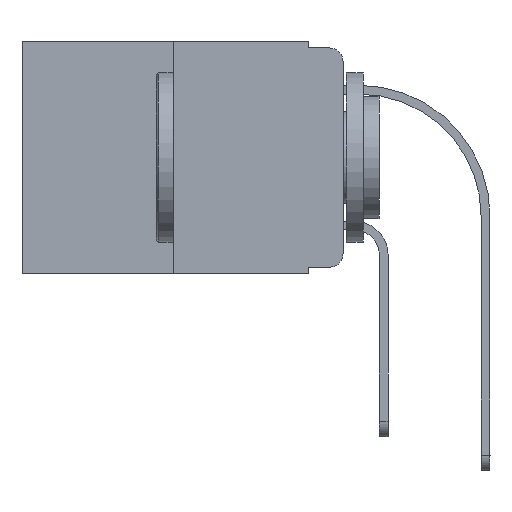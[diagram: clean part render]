
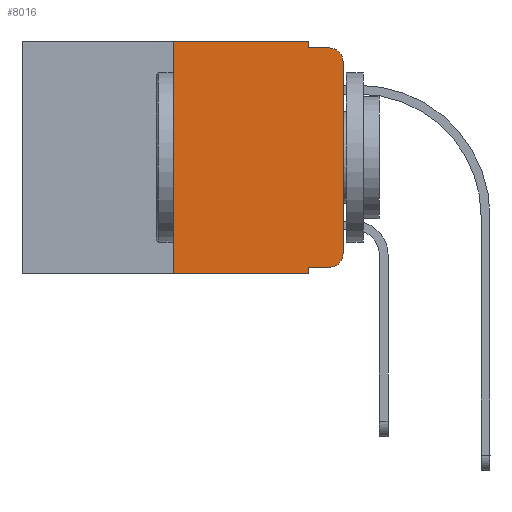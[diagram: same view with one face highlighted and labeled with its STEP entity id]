
A CAD part, left-side view. The second image highlights one B-rep face of the part: STEP entity #8016.
In plain terms, the highlighted planar face has unit normal (-1, 0, 0).
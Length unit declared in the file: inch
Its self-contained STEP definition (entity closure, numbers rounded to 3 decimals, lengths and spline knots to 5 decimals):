
#604 = ORIENTED_EDGE ( 'NONE', *, *, #14127, .T. ) ;
#701 = VERTEX_POINT ( 'NONE', #3576 ) ;
#734 = DIRECTION ( 'NONE',  ( 0., -1., 0. ) ) ;
#1061 = VECTOR ( 'NONE', #15440, 39.37008 ) ;
#1544 = VERTEX_POINT ( 'NONE', #9399 ) ;
#1588 = VECTOR ( 'NONE', #6368, 39.37008 ) ;
#1651 = CARTESIAN_POINT ( 'NONE',  ( 0., 0., 0. ) ) ;
#1813 = LINE ( 'NONE', #12721, #18763 ) ;
#1842 = EDGE_CURVE ( 'NONE', #6208, #13516, #20050, .T. ) ;
#2328 = CARTESIAN_POINT ( 'NONE',  ( 0., 0.473, 0. ) ) ;
#2438 = DIRECTION ( 'NONE',  ( 1., 0., 0. ) ) ;
#2763 = AXIS2_PLACEMENT_3D ( 'NONE', #20261, #9023, #14079 ) ;
#2826 = EDGE_LOOP ( 'NONE', ( #6298, #4714, #5255, #6037, #14143, #20571, #604, #4572, #17367, #7953 ) ) ;
#2975 = CARTESIAN_POINT ( 'NONE',  ( 0., 0.051, -0.01 ) ) ;
#3067 = LINE ( 'NONE', #9663, #14482 ) ;
#3576 = CARTESIAN_POINT ( 'NONE',  ( 0., 0.25, -0.343 ) ) ;
#4572 = ORIENTED_EDGE ( 'NONE', *, *, #15719, .F. ) ;
#4573 = EDGE_CURVE ( 'NONE', #1544, #17947, #17360, .T. ) ;
#4714 = ORIENTED_EDGE ( 'NONE', *, *, #16092, .T. ) ;
#4744 = DIRECTION ( 'NONE',  ( 0., -1., 0. ) ) ;
#4976 = LINE ( 'NONE', #14415, #9461 ) ;
#5255 = ORIENTED_EDGE ( 'NONE', *, *, #11853, .F. ) ;
#5357 = CARTESIAN_POINT ( 'NONE',  ( 0., 0.473, 0. ) ) ;
#5797 = DIRECTION ( 'NONE',  ( 0., 0., -1. ) ) ;
#5975 = EDGE_CURVE ( 'NONE', #14881, #17803, #6157, .T. ) ;
#5980 = CARTESIAN_POINT ( 'NONE',  ( 0., 0.02, -0.03 ) ) ;
#6037 = ORIENTED_EDGE ( 'NONE', *, *, #4573, .F. ) ;
#6157 = LINE ( 'NONE', #1651, #1588 ) ;
#6208 = VERTEX_POINT ( 'NONE', #13477 ) ;
#6277 = VERTEX_POINT ( 'NONE', #12013 ) ;
#6298 = ORIENTED_EDGE ( 'NONE', *, *, #5975, .T. ) ;
#6368 = DIRECTION ( 'NONE',  ( 0., 0., 1. ) ) ;
#7904 = VECTOR ( 'NONE', #15591, 39.37008 ) ;
#7953 = ORIENTED_EDGE ( 'NONE', *, *, #19572, .T. ) ;
#8016 = ADVANCED_FACE ( 'NONE', ( #12410 ), #19958, .F. ) ;
#8118 = CIRCLE ( 'NONE', #12814, 0.02 ) ;
#9023 = DIRECTION ( 'NONE',  ( -1., 0., 0. ) ) ;
#9180 = CARTESIAN_POINT ( 'NONE',  ( 0., 0.051, 0. ) ) ;
#9399 = CARTESIAN_POINT ( 'NONE',  ( 0., 0.051, 0. ) ) ;
#9461 = VECTOR ( 'NONE', #9682, 39.37008 ) ;
#9663 = CARTESIAN_POINT ( 'NONE',  ( 0., 0.051, 0. ) ) ;
#9682 = DIRECTION ( 'NONE',  ( 0., -1., 0. ) ) ;
#10617 = CARTESIAN_POINT ( 'NONE',  ( 0., 0.051, -0.333 ) ) ;
#11186 = DIRECTION ( 'NONE',  ( 0., 0., 1. ) ) ;
#11853 = EDGE_CURVE ( 'NONE', #17947, #14939, #1813, .T. ) ;
#12013 = CARTESIAN_POINT ( 'NONE',  ( 0., 0.25, 0. ) ) ;
#12074 = EDGE_CURVE ( 'NONE', #6277, #1544, #15108, .T. ) ;
#12252 = CARTESIAN_POINT ( 'NONE',  ( 0., 0., -0.313 ) ) ;
#12410 = FACE_OUTER_BOUND ( 'NONE', #2826, .T. ) ;
#12683 = CARTESIAN_POINT ( 'NONE',  ( 0., 0.051, -0.343 ) ) ;
#12721 = CARTESIAN_POINT ( 'NONE',  ( 0., 0.051, -0.01 ) ) ;
#12814 = AXIS2_PLACEMENT_3D ( 'NONE', #5980, #18566, #18769 ) ;
#13069 = LINE ( 'NONE', #19146, #18872 ) ;
#13326 = VECTOR ( 'NONE', #734, 39.37008 ) ;
#13477 = CARTESIAN_POINT ( 'NONE',  ( 0., 0.051, -0.333 ) ) ;
#13516 = VERTEX_POINT ( 'NONE', #18318 ) ;
#14079 = DIRECTION ( 'NONE',  ( 0., 0., -1. ) ) ;
#14127 = EDGE_CURVE ( 'NONE', #701, #18894, #4976, .T. ) ;
#14143 = ORIENTED_EDGE ( 'NONE', *, *, #12074, .F. ) ;
#14415 = CARTESIAN_POINT ( 'NONE',  ( 0., 0.473, -0.343 ) ) ;
#14482 = VECTOR ( 'NONE', #20476, 39.37008 ) ;
#14881 = VERTEX_POINT ( 'NONE', #12252 ) ;
#14939 = VERTEX_POINT ( 'NONE', #19467 ) ;
#15108 = LINE ( 'NONE', #5357, #13326 ) ;
#15234 = AXIS2_PLACEMENT_3D ( 'NONE', #2328, #2438, #5797 ) ;
#15440 = DIRECTION ( 'NONE',  ( 0., -1., 0. ) ) ;
#15591 = DIRECTION ( 'NONE',  ( 0., 0., -1. ) ) ;
#15719 = EDGE_CURVE ( 'NONE', #6208, #18894, #3067, .T. ) ;
#16092 = EDGE_CURVE ( 'NONE', #17803, #14939, #8118, .T. ) ;
#17360 = LINE ( 'NONE', #9180, #7904 ) ;
#17367 = ORIENTED_EDGE ( 'NONE', *, *, #1842, .T. ) ;
#17505 = EDGE_CURVE ( 'NONE', #701, #6277, #13069, .T. ) ;
#17803 = VERTEX_POINT ( 'NONE', #20070 ) ;
#17947 = VERTEX_POINT ( 'NONE', #2975 ) ;
#18153 = CIRCLE ( 'NONE', #2763, 0.02 ) ;
#18318 = CARTESIAN_POINT ( 'NONE',  ( 0., 0.02, -0.333 ) ) ;
#18566 = DIRECTION ( 'NONE',  ( -1., 0., 0. ) ) ;
#18763 = VECTOR ( 'NONE', #4744, 39.37008 ) ;
#18769 = DIRECTION ( 'NONE',  ( 0., 0., -1. ) ) ;
#18872 = VECTOR ( 'NONE', #11186, 39.37008 ) ;
#18894 = VERTEX_POINT ( 'NONE', #12683 ) ;
#19146 = CARTESIAN_POINT ( 'NONE',  ( 0., 0.25, 0. ) ) ;
#19467 = CARTESIAN_POINT ( 'NONE',  ( 0., 0.02, -0.01 ) ) ;
#19572 = EDGE_CURVE ( 'NONE', #13516, #14881, #18153, .T. ) ;
#19958 = PLANE ( 'NONE',  #15234 ) ;
#20050 = LINE ( 'NONE', #10617, #1061 ) ;
#20070 = CARTESIAN_POINT ( 'NONE',  ( 0., 0., -0.03 ) ) ;
#20261 = CARTESIAN_POINT ( 'NONE',  ( 0., 0.02, -0.313 ) ) ;
#20476 = DIRECTION ( 'NONE',  ( 0., 0., -1. ) ) ;
#20571 = ORIENTED_EDGE ( 'NONE', *, *, #17505, .F. ) ;
